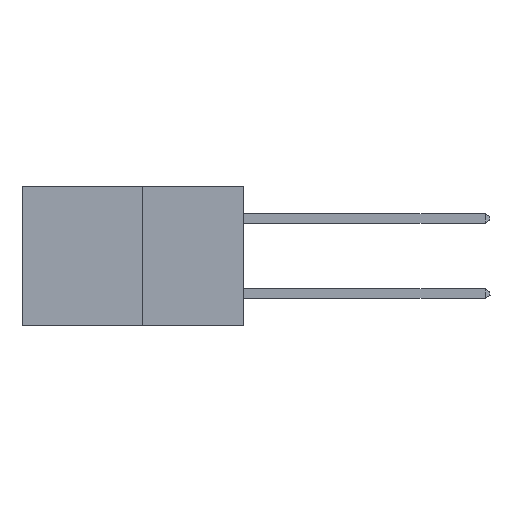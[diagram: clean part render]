
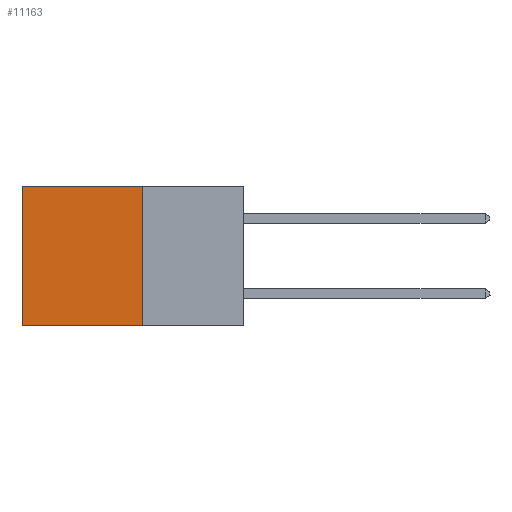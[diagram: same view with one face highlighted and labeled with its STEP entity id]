
A CAD part, left-side view. The second image highlights one B-rep face of the part: STEP entity #11163.
In plain terms, the highlighted planar face has unit normal (-1, 0, 0).
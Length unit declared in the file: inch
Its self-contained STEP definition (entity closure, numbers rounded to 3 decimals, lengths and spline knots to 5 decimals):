
#47 = VERTEX_POINT ( 'NONE', #2113 ) ;
#789 = CARTESIAN_POINT ( 'NONE',  ( 0.277, 0.27, -0.37 ) ) ;
#980 = VERTEX_POINT ( 'NONE', #5907 ) ;
#1651 = DIRECTION ( 'NONE',  ( 0., 1., 0. ) ) ;
#1849 = DIRECTION ( 'NONE',  ( 0., 0., -1. ) ) ;
#1948 = DIRECTION ( 'NONE',  ( 0., 0., -1. ) ) ;
#2070 = CARTESIAN_POINT ( 'NONE',  ( 0.277, 0.27, -0.37 ) ) ;
#2113 = CARTESIAN_POINT ( 'NONE',  ( 0.277, 0.27, -0.37 ) ) ;
#2823 = EDGE_CURVE ( 'NONE', #3980, #980, #8869, .T. ) ;
#3264 = DIRECTION ( 'NONE',  ( 0., 0., -1. ) ) ;
#3412 = VECTOR ( 'NONE', #3264, 39.37008 ) ;
#3512 = VECTOR ( 'NONE', #1651, 39.37008 ) ;
#3820 = EDGE_CURVE ( 'NONE', #3980, #47, #8844, .T. ) ;
#3904 = ORIENTED_EDGE ( 'NONE', *, *, #3820, .F. ) ;
#3980 = VERTEX_POINT ( 'NONE', #5825 ) ;
#4033 = VERTEX_POINT ( 'NONE', #13082 ) ;
#4579 = EDGE_CURVE ( 'NONE', #47, #4033, #12788, .T. ) ;
#5579 = VECTOR ( 'NONE', #1948, 39.37008 ) ;
#5616 = AXIS2_PLACEMENT_3D ( 'NONE', #789, #7905, #1849 ) ;
#5825 = CARTESIAN_POINT ( 'NONE',  ( 0.277, 0.27, 0. ) ) ;
#5907 = CARTESIAN_POINT ( 'NONE',  ( 0.277, 0.59, 0. ) ) ;
#6424 = EDGE_CURVE ( 'NONE', #980, #4033, #11492, .T. ) ;
#7016 = ORIENTED_EDGE ( 'NONE', *, *, #6424, .T. ) ;
#7201 = EDGE_LOOP ( 'NONE', ( #7016, #9586, #3904, #11327 ) ) ;
#7335 = CARTESIAN_POINT ( 'NONE',  ( 0.277, 0.27, 0. ) ) ;
#7718 = VECTOR ( 'NONE', #9724, 39.37008 ) ;
#7905 = DIRECTION ( 'NONE',  ( 1., 0., 0. ) ) ;
#8260 = CARTESIAN_POINT ( 'NONE',  ( 0.277, 0.59, -0.37 ) ) ;
#8844 = LINE ( 'NONE', #2070, #5579 ) ;
#8869 = LINE ( 'NONE', #7335, #3512 ) ;
#9586 = ORIENTED_EDGE ( 'NONE', *, *, #4579, .F. ) ;
#9588 = CARTESIAN_POINT ( 'NONE',  ( 0.277, 0.27, -0.37 ) ) ;
#9724 = DIRECTION ( 'NONE',  ( 0., 1., 0. ) ) ;
#11163 = ADVANCED_FACE ( 'NONE', ( #12834 ), #12964, .F. ) ;
#11327 = ORIENTED_EDGE ( 'NONE', *, *, #2823, .T. ) ;
#11492 = LINE ( 'NONE', #8260, #3412 ) ;
#12788 = LINE ( 'NONE', #9588, #7718 ) ;
#12834 = FACE_OUTER_BOUND ( 'NONE', #7201, .T. ) ;
#12964 = PLANE ( 'NONE',  #5616 ) ;
#13082 = CARTESIAN_POINT ( 'NONE',  ( 0.277, 0.59, -0.37 ) ) ;
